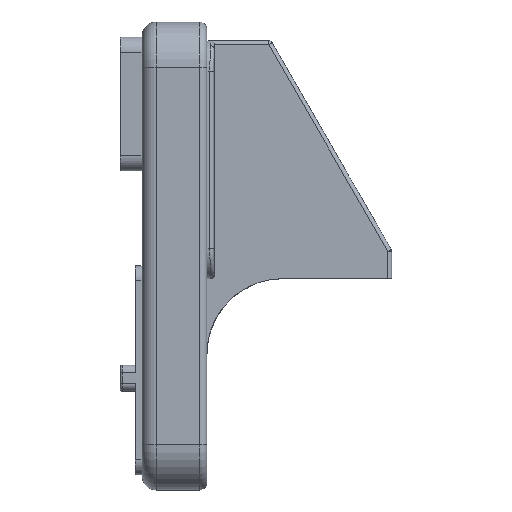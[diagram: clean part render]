
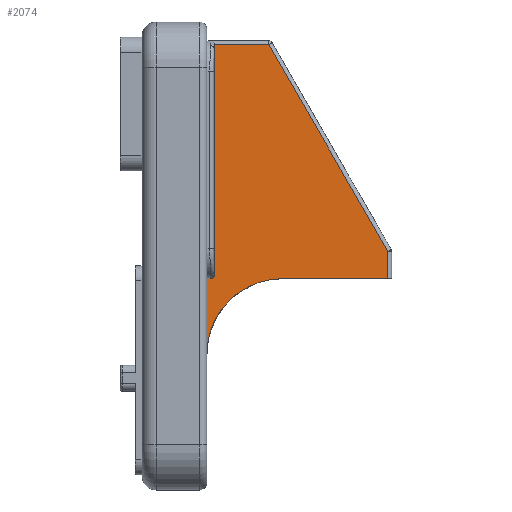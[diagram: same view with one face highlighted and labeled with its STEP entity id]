
A CAD part, left-side view. The second image highlights one B-rep face of the part: STEP entity #2074.
In plain terms, the highlighted planar face has unit normal (-1, 0, 0).
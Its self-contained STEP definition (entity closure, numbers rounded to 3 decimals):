
#57=B_SPLINE_CURVE_WITH_KNOTS('',3,(#3314,#3315,#3316,#3317,#3318,#3319,
#3320,#3321,#3322,#3323,#3324,#3325,#3326,#3327,#3328,#3329),
 .UNSPECIFIED.,.F.,.F.,(4,2,2,2,2,2,2,4),(0.,0.043,0.061,
0.073,0.085,0.103,0.138,
0.148),.UNSPECIFIED.);
#129=PLANE('',#2342);
#249=FACE_OUTER_BOUND('',#384,.T.);
#384=EDGE_LOOP('',(#1861,#1862,#1863,#1864,#1865,#1866,#1867,#1868,#1869,
#1870,#1871));
#417=LINE('',#3437,#553);
#428=LINE('',#3495,#564);
#497=LINE('',#3971,#633);
#503=LINE('',#4161,#639);
#518=LINE('',#4198,#654);
#524=LINE('',#4219,#660);
#525=LINE('',#4222,#661);
#553=VECTOR('',#2445,10.);
#564=VECTOR('',#2492,10.);
#633=VECTOR('',#2859,10.);
#639=VECTOR('',#2905,10.);
#654=VECTOR('',#2952,10.);
#660=VECTOR('',#2978,10.);
#661=VECTOR('',#2983,10.);
#693=CIRCLE('',#2134,10.);
#698=CIRCLE('',#2142,10.);
#772=CIRCLE('',#2283,0.5);
#842=VERTEX_POINT('',#3312);
#843=VERTEX_POINT('',#3313);
#848=VERTEX_POINT('',#3434);
#849=VERTEX_POINT('',#3436);
#864=VERTEX_POINT('',#3483);
#868=VERTEX_POINT('',#3493);
#948=VERTEX_POINT('',#3914);
#949=VERTEX_POINT('',#3916);
#953=VERTEX_POINT('',#3963);
#976=VERTEX_POINT('',#4196);
#981=VERTEX_POINT('',#4218);
#1035=EDGE_CURVE('',#842,#843,#57,.T.);
#1046=EDGE_CURVE('',#848,#849,#417,.T.);
#1059=EDGE_CURVE('',#843,#848,#693,.T.);
#1067=EDGE_CURVE('',#864,#842,#698,.T.);
#1072=EDGE_CURVE('',#868,#864,#428,.T.);
#1211=EDGE_CURVE('',#948,#949,#772,.F.);
#1225=EDGE_CURVE('',#949,#953,#497,.T.);
#1249=EDGE_CURVE('',#849,#948,#503,.T.);
#1268=EDGE_CURVE('',#953,#976,#518,.T.);
#1278=EDGE_CURVE('',#976,#981,#524,.T.);
#1280=EDGE_CURVE('',#981,#868,#525,.T.);
#1861=ORIENTED_EDGE('',*,*,#1035,.F.);
#1862=ORIENTED_EDGE('',*,*,#1067,.F.);
#1863=ORIENTED_EDGE('',*,*,#1072,.F.);
#1864=ORIENTED_EDGE('',*,*,#1280,.F.);
#1865=ORIENTED_EDGE('',*,*,#1278,.F.);
#1866=ORIENTED_EDGE('',*,*,#1268,.F.);
#1867=ORIENTED_EDGE('',*,*,#1225,.F.);
#1868=ORIENTED_EDGE('',*,*,#1211,.F.);
#1869=ORIENTED_EDGE('',*,*,#1249,.F.);
#1870=ORIENTED_EDGE('',*,*,#1046,.F.);
#1871=ORIENTED_EDGE('',*,*,#1059,.F.);
#2074=ADVANCED_FACE('',(#249),#129,.T.);
#2134=AXIS2_PLACEMENT_3D('',#3462,#2465,#2466);
#2142=AXIS2_PLACEMENT_3D('',#3485,#2482,#2483);
#2283=AXIS2_PLACEMENT_3D('',#3917,#2829,#2830);
#2342=AXIS2_PLACEMENT_3D('',#4221,#2981,#2982);
#2445=DIRECTION('',(0.,0.,1.));
#2465=DIRECTION('center_axis',(-1.,0.,0.));
#2466=DIRECTION('ref_axis',(0.,0.707,0.707));
#2482=DIRECTION('center_axis',(-1.,0.,0.));
#2483=DIRECTION('ref_axis',(0.,0.707,0.707));
#2492=DIRECTION('',(0.,1.,0.));
#2829=DIRECTION('center_axis',(1.,0.,0.));
#2830=DIRECTION('ref_axis',(0.,-0.707,-0.707));
#2859=DIRECTION('',(0.,0.,1.));
#2905=DIRECTION('',(0.,-1.,0.));
#2952=DIRECTION('',(0.,-1.,0.));
#2978=DIRECTION('',(0.,-0.499,-0.866));
#2981=DIRECTION('center_axis',(-1.,0.,0.));
#2982=DIRECTION('ref_axis',(0.,-1.,0.));
#2983=DIRECTION('',(0.,0.,-1.));
#3312=CARTESIAN_POINT('',(78.925,-1.852,-55.437));
#3313=CARTESIAN_POINT('',(78.925,-1.28,-56.789));
#3314=CARTESIAN_POINT('Ctrl Pts',(78.925,-1.852,-55.437));
#3315=CARTESIAN_POINT('Ctrl Pts',(78.925,-1.787,-55.564));
#3316=CARTESIAN_POINT('Ctrl Pts',(78.925,-1.725,-55.689));
#3317=CARTESIAN_POINT('Ctrl Pts',(78.925,-1.64,-55.872));
#3318=CARTESIAN_POINT('Ctrl Pts',(78.925,-1.615,-55.927));
#3319=CARTESIAN_POINT('Ctrl Pts',(78.925,-1.575,-56.019));
#3320=CARTESIAN_POINT('Ctrl Pts',(78.925,-1.558,-56.057));
#3321=CARTESIAN_POINT('Ctrl Pts',(78.925,-1.526,-56.133));
#3322=CARTESIAN_POINT('Ctrl Pts',(78.925,-1.51,-56.171));
#3323=CARTESIAN_POINT('Ctrl Pts',(78.925,-1.473,-56.263));
#3324=CARTESIAN_POINT('Ctrl Pts',(78.925,-1.452,-56.316));
#3325=CARTESIAN_POINT('Ctrl Pts',(78.925,-1.388,-56.481));
#3326=CARTESIAN_POINT('Ctrl Pts',(78.925,-1.349,-56.59));
#3327=CARTESIAN_POINT('Ctrl Pts',(78.925,-1.3,-56.731));
#3328=CARTESIAN_POINT('Ctrl Pts',(78.925,-1.29,-56.76));
#3329=CARTESIAN_POINT('Ctrl Pts',(78.925,-1.28,-56.789));
#3434=CARTESIAN_POINT('',(78.925,-0.75,-60.001));
#3436=CARTESIAN_POINT('',(78.925,-0.75,-50.));
#3437=CARTESIAN_POINT('',(78.925,-0.75,-48.5));
#3462=CARTESIAN_POINT('Origin',(78.925,-10.75,-60.001));
#3483=CARTESIAN_POINT('',(78.925,-10.75,-50.001));
#3485=CARTESIAN_POINT('Origin',(78.925,-10.75,-60.001));
#3493=CARTESIAN_POINT('',(78.925,-24.725,-50.001));
#3495=CARTESIAN_POINT('',(78.925,-24.725,-50.001));
#3914=CARTESIAN_POINT('',(78.925,-1.225,-50.));
#3916=CARTESIAN_POINT('',(78.925,-1.725,-49.5));
#3917=CARTESIAN_POINT('Origin',(78.925,-1.225,-49.5));
#3963=CARTESIAN_POINT('',(78.925,-1.725,-19.));
#3971=CARTESIAN_POINT('',(78.925,-1.725,-50.));
#4161=CARTESIAN_POINT('',(78.925,-15.163,-50.));
#4196=CARTESIAN_POINT('',(78.925,-8.936,-19.));
#4198=CARTESIAN_POINT('',(78.925,-3.663,-19.));
#4218=CARTESIAN_POINT('',(78.925,-24.725,-46.384));
#4219=CARTESIAN_POINT('',(78.925,-22.672,-42.822));
#4221=CARTESIAN_POINT('Origin',(78.925,-1.725,-50.));
#4222=CARTESIAN_POINT('',(78.925,-24.725,-50.));
